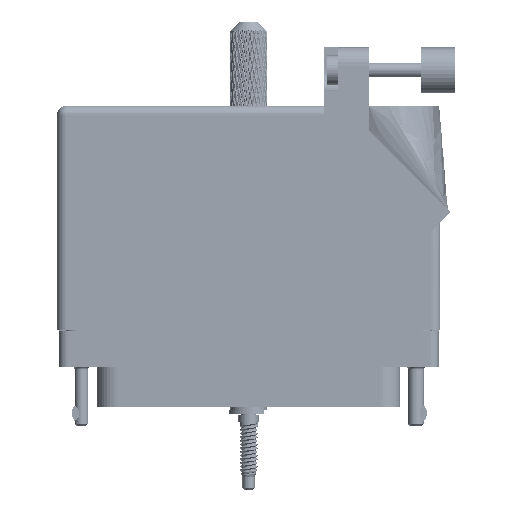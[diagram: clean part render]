
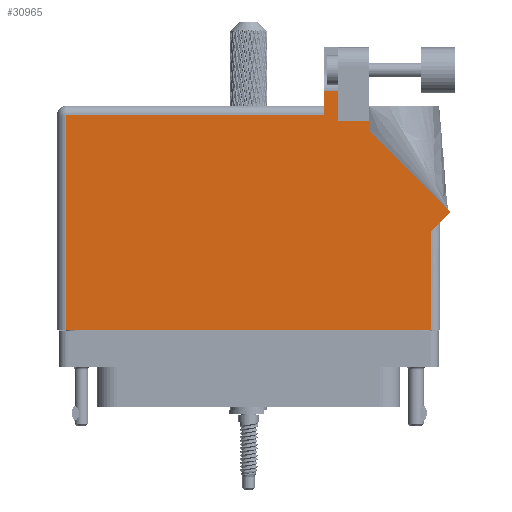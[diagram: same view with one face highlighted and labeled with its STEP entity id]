
A CAD part, front view. The second image highlights one B-rep face of the part: STEP entity #30965.
In plain terms, the highlighted face is planar.
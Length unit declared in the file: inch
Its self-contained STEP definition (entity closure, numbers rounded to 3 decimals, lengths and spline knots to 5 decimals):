
#2058 = VERTEX_POINT ( 'NONE', #92409 ) ;
#5162 = CARTESIAN_POINT ( 'NONE',  ( 0.513, 1.368, 0.455 ) ) ;
#6587 = PLANE ( 'NONE',  #33125 ) ;
#7129 = LINE ( 'NONE', #55823, #83751 ) ;
#8097 = DIRECTION ( 'NONE',  ( 0., 1., 0. ) ) ;
#9400 = ORIENTED_EDGE ( 'NONE', *, *, #60389, .T. ) ;
#11815 = EDGE_CURVE ( 'NONE', #45410, #52332, #21181, .T. ) ;
#13859 = EDGE_CURVE ( 'NONE', #37983, #56243, #119023, .T. ) ;
#14185 = CARTESIAN_POINT ( 'NONE',  ( 0.513, 1.5315, 0.455 ) ) ;
#14446 = DIRECTION ( 'NONE',  ( 0., 1., 0. ) ) ;
#15285 = LINE ( 'NONE', #28315, #90431 ) ;
#15979 = CARTESIAN_POINT ( 'NONE',  ( 0.513, 1.43, 0.455 ) ) ;
#18464 = EDGE_CURVE ( 'NONE', #100612, #2058, #15285, .T. ) ;
#18600 = LINE ( 'NONE', #35541, #119899 ) ;
#20218 = CARTESIAN_POINT ( 'NONE',  ( 0.607, 1.33, 0.455 ) ) ;
#21181 = LINE ( 'NONE', #39636, #119397 ) ;
#24039 = CARTESIAN_POINT ( 'NONE',  ( 0.82, 1.33, 0.455 ) ) ;
#28315 = CARTESIAN_POINT ( 'NONE',  ( 1.37671, 0.70771, 0.455 ) ) ;
#28865 = CARTESIAN_POINT ( 'NONE',  ( 0.82, 1.33, 0.455 ) ) ;
#30925 = VECTOR ( 'NONE', #14446, 39.37008 ) ;
#30965 = ADVANCED_FACE ( 'NONE', ( #111417 ), #6587, .F. ) ;
#33125 = AXIS2_PLACEMENT_3D ( 'NONE', #63202, #46067, #65326 ) ;
#33841 = LINE ( 'NONE', #85685, #119794 ) ;
#35151 = DIRECTION ( 'NONE',  ( 0., 1., 0. ) ) ;
#35541 = CARTESIAN_POINT ( 'NONE',  ( 1.306, 0.637, 0.455 ) ) ;
#36123 = DIRECTION ( 'NONE',  ( 0., -1., 0. ) ) ;
#37983 = VERTEX_POINT ( 'NONE', #28865 ) ;
#39288 = VECTOR ( 'NONE', #53250, 39.37008 ) ;
#39636 = CARTESIAN_POINT ( 'NONE',  ( -1.306, 1.368, 0.455 ) ) ;
#41992 = VERTEX_POINT ( 'NONE', #101575 ) ;
#44842 = EDGE_CURVE ( 'NONE', #97605, #41992, #67209, .T. ) ;
#45410 = VERTEX_POINT ( 'NONE', #5162 ) ;
#46067 = DIRECTION ( 'NONE',  ( 0., 0., -1. ) ) ;
#49441 = ORIENTED_EDGE ( 'NONE', *, *, #11815, .T. ) ;
#52301 = VERTEX_POINT ( 'NONE', #71271 ) ;
#52332 = VERTEX_POINT ( 'NONE', #91802 ) ;
#53250 = DIRECTION ( 'NONE',  ( -1., 0., 0. ) ) ;
#53358 = ORIENTED_EDGE ( 'NONE', *, *, #13859, .T. ) ;
#55060 = DIRECTION ( 'NONE',  ( 1., 0., 0. ) ) ;
#55823 = CARTESIAN_POINT ( 'NONE',  ( -1.244, -0.1, 0.455 ) ) ;
#56243 = VERTEX_POINT ( 'NONE', #20218 ) ;
#57748 = CARTESIAN_POINT ( 'NONE',  ( -1.244, -0.1, 0.455 ) ) ;
#60389 = EDGE_CURVE ( 'NONE', #126376, #45410, #106197, .T. ) ;
#61016 = ORIENTED_EDGE ( 'NONE', *, *, #94669, .T. ) ;
#63202 = CARTESIAN_POINT ( 'NONE',  ( -1.306, 1.43, 0.455 ) ) ;
#63889 = VECTOR ( 'NONE', #35151, 39.37008 ) ;
#65326 = DIRECTION ( 'NONE',  ( -1., 0., 0. ) ) ;
#67209 = LINE ( 'NONE', #105166, #94914 ) ;
#67514 = ORIENTED_EDGE ( 'NONE', *, *, #120418, .T. ) ;
#67630 = ORIENTED_EDGE ( 'NONE', *, *, #101456, .T. ) ;
#68514 = ORIENTED_EDGE ( 'NONE', *, *, #44842, .T. ) ;
#71186 = ORIENTED_EDGE ( 'NONE', *, *, #18464, .T. ) ;
#71271 = CARTESIAN_POINT ( 'NONE',  ( 1.244, 0.575, 0.455 ) ) ;
#74441 = EDGE_CURVE ( 'NONE', #52332, #97605, #7129, .T. ) ;
#78516 = EDGE_LOOP ( 'NONE', ( #61016, #67514, #9400, #49441, #112588, #68514, #127273, #119394, #71186, #67630, #53358 ) ) ;
#79039 = EDGE_CURVE ( 'NONE', #52301, #100612, #18600, .T. ) ;
#83570 = DIRECTION ( 'NONE',  ( 0.707, 0.707, 0. ) ) ;
#83751 = VECTOR ( 'NONE', #84530, 39.37008 ) ;
#84530 = DIRECTION ( 'NONE',  ( 0., -1., 0. ) ) ;
#85685 = CARTESIAN_POINT ( 'NONE',  ( 1.244, 0.637, 0.455 ) ) ;
#90431 = VECTOR ( 'NONE', #126532, 39.37008 ) ;
#91354 = CARTESIAN_POINT ( 'NONE',  ( 0.607, 1.5315, 0.455 ) ) ;
#91802 = CARTESIAN_POINT ( 'NONE',  ( -1.244, 1.368, 0.455 ) ) ;
#92409 = CARTESIAN_POINT ( 'NONE',  ( 0.82, 1.26442, 0.455 ) ) ;
#93039 = CARTESIAN_POINT ( 'NONE',  ( 0.607, 1.33, 0.455 ) ) ;
#94669 = EDGE_CURVE ( 'NONE', #56243, #105101, #108271, .T. ) ;
#94914 = VECTOR ( 'NONE', #55060, 39.37008 ) ;
#97605 = VERTEX_POINT ( 'NONE', #57748 ) ;
#100612 = VERTEX_POINT ( 'NONE', #125784 ) ;
#101456 = EDGE_CURVE ( 'NONE', #2058, #37983, #116814, .T. ) ;
#101575 = CARTESIAN_POINT ( 'NONE',  ( 1.244, -0.1, 0.455 ) ) ;
#102264 = EDGE_CURVE ( 'NONE', #41992, #52301, #33841, .T. ) ;
#105101 = VERTEX_POINT ( 'NONE', #91354 ) ;
#105166 = CARTESIAN_POINT ( 'NONE',  ( -1.306, -0.1, 0.455 ) ) ;
#106197 = LINE ( 'NONE', #15979, #123104 ) ;
#108271 = LINE ( 'NONE', #93039, #63889 ) ;
#109869 = DIRECTION ( 'NONE',  ( -1., 0., 0. ) ) ;
#111417 = FACE_OUTER_BOUND ( 'NONE', #78516, .T. ) ;
#111890 = DIRECTION ( 'NONE',  ( -1., 0., 0. ) ) ;
#111947 = CARTESIAN_POINT ( 'NONE',  ( 0.93777, 1.5315, 0.455 ) ) ;
#112588 = ORIENTED_EDGE ( 'NONE', *, *, #74441, .T. ) ;
#116060 = LINE ( 'NONE', #111947, #39288 ) ;
#116814 = LINE ( 'NONE', #122099, #30925 ) ;
#119023 = LINE ( 'NONE', #24039, #122104 ) ;
#119394 = ORIENTED_EDGE ( 'NONE', *, *, #79039, .T. ) ;
#119397 = VECTOR ( 'NONE', #109869, 39.37008 ) ;
#119794 = VECTOR ( 'NONE', #8097, 39.37008 ) ;
#119899 = VECTOR ( 'NONE', #83570, 39.37008 ) ;
#120418 = EDGE_CURVE ( 'NONE', #105101, #126376, #116060, .T. ) ;
#122099 = CARTESIAN_POINT ( 'NONE',  ( 0.82, 1.26442, 0.455 ) ) ;
#122104 = VECTOR ( 'NONE', #111890, 39.37008 ) ;
#123104 = VECTOR ( 'NONE', #36123, 39.37008 ) ;
#125784 = CARTESIAN_POINT ( 'NONE',  ( 1.37671, 0.70771, 0.455 ) ) ;
#126376 = VERTEX_POINT ( 'NONE', #14185 ) ;
#126532 = DIRECTION ( 'NONE',  ( -0.707, 0.707, 0. ) ) ;
#127273 = ORIENTED_EDGE ( 'NONE', *, *, #102264, .T. ) ;
